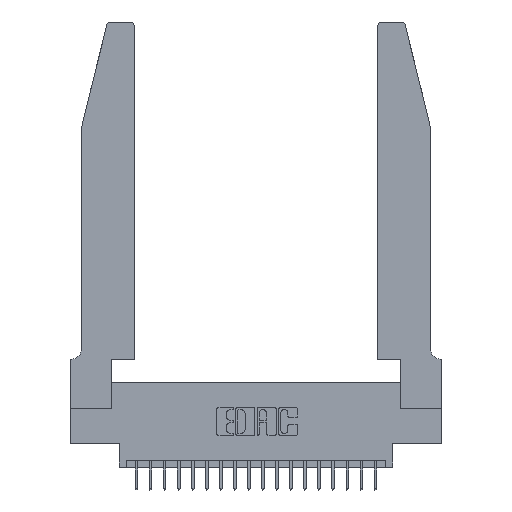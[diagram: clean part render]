
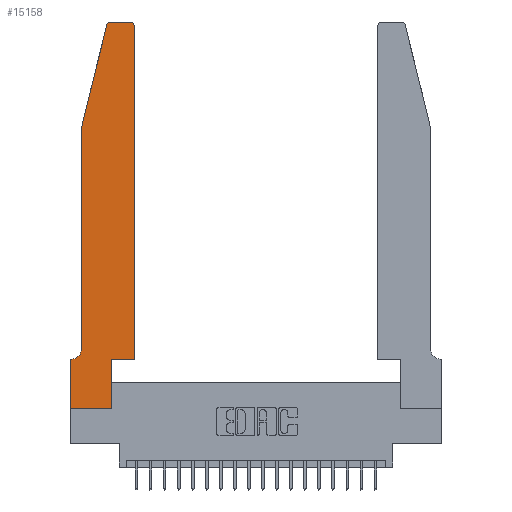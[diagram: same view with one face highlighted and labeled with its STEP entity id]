
A CAD part, top view. The second image highlights one B-rep face of the part: STEP entity #15158.
In plain terms, the highlighted planar face has unit normal (0, 0, 1).
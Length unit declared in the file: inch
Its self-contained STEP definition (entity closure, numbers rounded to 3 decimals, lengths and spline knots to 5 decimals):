
#446 = DIRECTION ( 'NONE',  ( 0., -1., 0. ) ) ;
#516 = EDGE_CURVE ( 'NONE', #1899, #6544, #627, .T. ) ;
#627 = LINE ( 'NONE', #5490, #14018 ) ;
#851 = LINE ( 'NONE', #8002, #22117 ) ;
#908 = VERTEX_POINT ( 'NONE', #16204 ) ;
#957 = VECTOR ( 'NONE', #6254, 39.37008 ) ;
#1386 = VERTEX_POINT ( 'NONE', #5461 ) ;
#1510 = CARTESIAN_POINT ( 'NONE',  ( 0.2865, 0.35, 0.37 ) ) ;
#1691 = LINE ( 'NONE', #18392, #18440 ) ;
#1811 = EDGE_CURVE ( 'NONE', #8741, #5938, #1691, .T. ) ;
#1872 = DIRECTION ( 'NONE',  ( 0., 0., -1. ) ) ;
#1899 = VERTEX_POINT ( 'NONE', #18636 ) ;
#2116 = EDGE_CURVE ( 'NONE', #15599, #5593, #851, .T. ) ;
#2281 = EDGE_CURVE ( 'NONE', #17648, #16022, #6991, .T. ) ;
#2973 = CARTESIAN_POINT ( 'NONE',  ( 0.0755, 2., 0.37 ) ) ;
#3248 = VECTOR ( 'NONE', #7677, 39.37008 ) ;
#3260 = EDGE_CURVE ( 'NONE', #6544, #15599, #8630, .T. ) ;
#3620 = AXIS2_PLACEMENT_3D ( 'NONE', #6223, #19815, #9742 ) ;
#4257 = CARTESIAN_POINT ( 'NONE',  ( 0.4505, 0.35, 0.37 ) ) ;
#4371 = CARTESIAN_POINT ( 'NONE',  ( 0.4205, 2.72, 0.37 ) ) ;
#4603 = DIRECTION ( 'NONE',  ( 0., 0., 1. ) ) ;
#4737 = VERTEX_POINT ( 'NONE', #21556 ) ;
#4782 = DIRECTION ( 'NONE',  ( 0., 0., 1. ) ) ;
#4783 = DIRECTION ( 'NONE',  ( 1., 0., 0. ) ) ;
#5461 = CARTESIAN_POINT ( 'NONE',  ( 0.4505, 0.35, 0.37 ) ) ;
#5490 = CARTESIAN_POINT ( 'NONE',  ( 0.0755, 0.35, 0.37 ) ) ;
#5590 = CARTESIAN_POINT ( 'NONE',  ( 0.2865, 0., 0.37 ) ) ;
#5593 = VERTEX_POINT ( 'NONE', #5590 ) ;
#5694 = LINE ( 'NONE', #11371, #957 ) ;
#5857 = ORIENTED_EDGE ( 'NONE', *, *, #8178, .T. ) ;
#5904 = CARTESIAN_POINT ( 'NONE',  ( 0.4505, 0.35, 0.37 ) ) ;
#5938 = VERTEX_POINT ( 'NONE', #2973 ) ;
#6223 = CARTESIAN_POINT ( 'NONE',  ( 0., 0.35, 0.37 ) ) ;
#6254 = DIRECTION ( 'NONE',  ( 0., 1., 0. ) ) ;
#6544 = VERTEX_POINT ( 'NONE', #18716 ) ;
#6664 = ORIENTED_EDGE ( 'NONE', *, *, #14064, .T. ) ;
#6891 = LINE ( 'NONE', #4257, #19904 ) ;
#6991 = CIRCLE ( 'NONE', #9120, 0.03 ) ;
#7298 = FACE_OUTER_BOUND ( 'NONE', #22119, .T. ) ;
#7493 = EDGE_CURVE ( 'NONE', #5593, #18374, #5694, .T. ) ;
#7554 = CARTESIAN_POINT ( 'NONE',  ( 0.0755, 2., 0.37 ) ) ;
#7677 = DIRECTION ( 'NONE',  ( 0., 1., 0. ) ) ;
#8002 = CARTESIAN_POINT ( 'NONE',  ( 0., 0., 0.37 ) ) ;
#8178 = EDGE_CURVE ( 'NONE', #16022, #908, #11635, .T. ) ;
#8550 = EDGE_CURVE ( 'NONE', #4737, #1899, #8700, .T. ) ;
#8554 = ORIENTED_EDGE ( 'NONE', *, *, #3260, .T. ) ;
#8630 = LINE ( 'NONE', #20874, #21564 ) ;
#8700 = CIRCLE ( 'NONE', #20634, 0.07 ) ;
#8740 = ORIENTED_EDGE ( 'NONE', *, *, #2116, .T. ) ;
#8741 = VERTEX_POINT ( 'NONE', #12744 ) ;
#9120 = AXIS2_PLACEMENT_3D ( 'NONE', #4371, #4603, #4783 ) ;
#9256 = CARTESIAN_POINT ( 'NONE',  ( 0., 0., 0.37 ) ) ;
#9742 = DIRECTION ( 'NONE',  ( 1., 0., 0. ) ) ;
#11371 = CARTESIAN_POINT ( 'NONE',  ( 0.2865, 0.35, 0.37 ) ) ;
#11635 = LINE ( 'NONE', #14660, #20069 ) ;
#11782 = EDGE_CURVE ( 'NONE', #18374, #1386, #6891, .T. ) ;
#12136 = ORIENTED_EDGE ( 'NONE', *, *, #8550, .T. ) ;
#12374 = CARTESIAN_POINT ( 'NONE',  ( 0.0055, 0.42, 0.37 ) ) ;
#12744 = CARTESIAN_POINT ( 'NONE',  ( 0.25487, 2.72718, 0.37 ) ) ;
#13084 = ORIENTED_EDGE ( 'NONE', *, *, #2281, .T. ) ;
#14018 = VECTOR ( 'NONE', #21844, 39.37008 ) ;
#14063 = DIRECTION ( 'NONE',  ( -1., 0., 0. ) ) ;
#14064 = EDGE_CURVE ( 'NONE', #908, #8741, #17978, .T. ) ;
#14468 = EDGE_CURVE ( 'NONE', #5938, #4737, #19007, .T. ) ;
#14512 = DIRECTION ( 'NONE',  ( 1., 0., 0. ) ) ;
#14516 = VECTOR ( 'NONE', #446, 39.37008 ) ;
#14554 = ORIENTED_EDGE ( 'NONE', *, *, #19720, .T. ) ;
#14660 = CARTESIAN_POINT ( 'NONE',  ( 0.2605, 2.75, 0.37 ) ) ;
#15087 = CARTESIAN_POINT ( 'NONE',  ( 0.284, 2.72, 0.37 ) ) ;
#15158 = ADVANCED_FACE ( 'NONE', ( #7298 ), #18118, .T. ) ;
#15240 = DIRECTION ( 'NONE',  ( 0., -1., 0. ) ) ;
#15599 = VERTEX_POINT ( 'NONE', #9256 ) ;
#16022 = VERTEX_POINT ( 'NONE', #17100 ) ;
#16204 = CARTESIAN_POINT ( 'NONE',  ( 0.284, 2.75, 0.37 ) ) ;
#16339 = DIRECTION ( 'NONE',  ( -1., 0., 0. ) ) ;
#16461 = LINE ( 'NONE', #5904, #3248 ) ;
#16760 = DIRECTION ( 'NONE',  ( 1., 0., 0. ) ) ;
#17100 = CARTESIAN_POINT ( 'NONE',  ( 0.4205, 2.75, 0.37 ) ) ;
#17648 = VERTEX_POINT ( 'NONE', #18744 ) ;
#17978 = CIRCLE ( 'NONE', #18008, 0.03 ) ;
#18008 = AXIS2_PLACEMENT_3D ( 'NONE', #15087, #4782, #16760 ) ;
#18118 = PLANE ( 'NONE',  #3620 ) ;
#18259 = DIRECTION ( 'NONE',  ( -0.239, -0.971, 0. ) ) ;
#18374 = VERTEX_POINT ( 'NONE', #1510 ) ;
#18392 = CARTESIAN_POINT ( 'NONE',  ( 0.0755, 2., 0.37 ) ) ;
#18440 = VECTOR ( 'NONE', #18259, 39.37008 ) ;
#18636 = CARTESIAN_POINT ( 'NONE',  ( 0.0055, 0.35, 0.37 ) ) ;
#18716 = CARTESIAN_POINT ( 'NONE',  ( 0., 0.35, 0.37 ) ) ;
#18724 = ORIENTED_EDGE ( 'NONE', *, *, #516, .T. ) ;
#18737 = DIRECTION ( 'NONE',  ( 1., 0., 0. ) ) ;
#18744 = CARTESIAN_POINT ( 'NONE',  ( 0.4505, 2.72, 0.37 ) ) ;
#19007 = LINE ( 'NONE', #7554, #14516 ) ;
#19648 = ORIENTED_EDGE ( 'NONE', *, *, #1811, .T. ) ;
#19720 = EDGE_CURVE ( 'NONE', #1386, #17648, #16461, .T. ) ;
#19799 = ORIENTED_EDGE ( 'NONE', *, *, #14468, .T. ) ;
#19815 = DIRECTION ( 'NONE',  ( 0., 0., 1. ) ) ;
#19904 = VECTOR ( 'NONE', #14512, 39.37008 ) ;
#20069 = VECTOR ( 'NONE', #16339, 39.37008 ) ;
#20508 = ORIENTED_EDGE ( 'NONE', *, *, #11782, .T. ) ;
#20634 = AXIS2_PLACEMENT_3D ( 'NONE', #12374, #1872, #14063 ) ;
#20874 = CARTESIAN_POINT ( 'NONE',  ( 0., 0., 0.37 ) ) ;
#21556 = CARTESIAN_POINT ( 'NONE',  ( 0.0755, 0.42, 0.37 ) ) ;
#21564 = VECTOR ( 'NONE', #15240, 39.37008 ) ;
#21844 = DIRECTION ( 'NONE',  ( -1., 0., 0. ) ) ;
#21965 = ORIENTED_EDGE ( 'NONE', *, *, #7493, .T. ) ;
#22117 = VECTOR ( 'NONE', #18737, 39.37008 ) ;
#22119 = EDGE_LOOP ( 'NONE', ( #5857, #6664, #19648, #19799, #12136, #18724, #8554, #8740, #21965, #20508, #14554, #13084 ) ) ;
